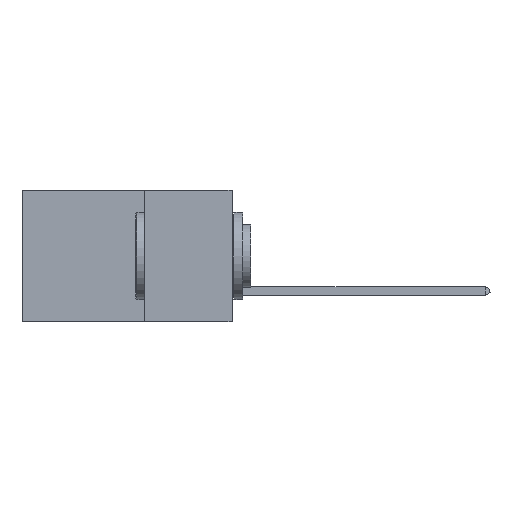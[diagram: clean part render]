
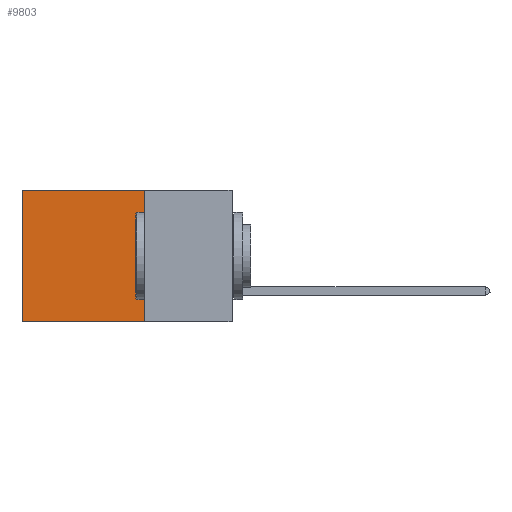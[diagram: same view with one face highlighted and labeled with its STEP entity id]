
A CAD part, left-side view. The second image highlights one B-rep face of the part: STEP entity #9803.
In plain terms, the highlighted planar face has unit normal (-1, 0, 0).
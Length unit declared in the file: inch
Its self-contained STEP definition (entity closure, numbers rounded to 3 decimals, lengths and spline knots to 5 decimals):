
#192 = LINE ( 'NONE', #19839, #1229 ) ;
#205 = EDGE_CURVE ( 'NONE', #3196, #5970, #15504, .T. ) ;
#1229 = VECTOR ( 'NONE', #13219, 39.37008 ) ;
#1980 = ORIENTED_EDGE ( 'NONE', *, *, #10326, .T. ) ;
#2737 = DIRECTION ( 'NONE',  ( 1., 0., 0. ) ) ;
#3146 = VECTOR ( 'NONE', #20060, 39.37008 ) ;
#3196 = VERTEX_POINT ( 'NONE', #13859 ) ;
#3802 = VERTEX_POINT ( 'NONE', #9001 ) ;
#3978 = DIRECTION ( 'NONE',  ( 0., 1., 0. ) ) ;
#4963 = ORIENTED_EDGE ( 'NONE', *, *, #5641, .T. ) ;
#5641 = EDGE_CURVE ( 'NONE', #3196, #3802, #7622, .T. ) ;
#5970 = VERTEX_POINT ( 'NONE', #16781 ) ;
#7522 = LINE ( 'NONE', #8488, #3146 ) ;
#7561 = DIRECTION ( 'NONE',  ( 0., 0., -1. ) ) ;
#7622 = LINE ( 'NONE', #12186, #21250 ) ;
#8222 = FACE_OUTER_BOUND ( 'NONE', #19397, .T. ) ;
#8359 = EDGE_CURVE ( 'NONE', #5970, #11813, #7522, .T. ) ;
#8488 = CARTESIAN_POINT ( 'NONE',  ( 0.2875, 0.25, -0.375 ) ) ;
#9001 = CARTESIAN_POINT ( 'NONE',  ( 0.2875, 0.6, 0. ) ) ;
#9803 = ADVANCED_FACE ( 'NONE', ( #8222 ), #10989, .F. ) ;
#10326 = EDGE_CURVE ( 'NONE', #3802, #11813, #192, .T. ) ;
#10989 = PLANE ( 'NONE',  #16988 ) ;
#11133 = CARTESIAN_POINT ( 'NONE',  ( 0.2875, 0.25, -0.375 ) ) ;
#11813 = VERTEX_POINT ( 'NONE', #14421 ) ;
#12186 = CARTESIAN_POINT ( 'NONE',  ( 0.2875, 0.25, 0. ) ) ;
#13219 = DIRECTION ( 'NONE',  ( 0., 0., -1. ) ) ;
#13859 = CARTESIAN_POINT ( 'NONE',  ( 0.2875, 0.25, 0. ) ) ;
#14421 = CARTESIAN_POINT ( 'NONE',  ( 0.2875, 0.6, -0.375 ) ) ;
#15504 = LINE ( 'NONE', #18904, #18321 ) ;
#16781 = CARTESIAN_POINT ( 'NONE',  ( 0.2875, 0.25, -0.375 ) ) ;
#16988 = AXIS2_PLACEMENT_3D ( 'NONE', #11133, #2737, #7561 ) ;
#17707 = ORIENTED_EDGE ( 'NONE', *, *, #205, .F. ) ;
#18321 = VECTOR ( 'NONE', #19105, 39.37008 ) ;
#18904 = CARTESIAN_POINT ( 'NONE',  ( 0.2875, 0.25, -0.375 ) ) ;
#19105 = DIRECTION ( 'NONE',  ( 0., 0., -1. ) ) ;
#19397 = EDGE_LOOP ( 'NONE', ( #1980, #21251, #17707, #4963 ) ) ;
#19839 = CARTESIAN_POINT ( 'NONE',  ( 0.2875, 0.6, -0.375 ) ) ;
#20060 = DIRECTION ( 'NONE',  ( 0., 1., 0. ) ) ;
#21250 = VECTOR ( 'NONE', #3978, 39.37008 ) ;
#21251 = ORIENTED_EDGE ( 'NONE', *, *, #8359, .F. ) ;
